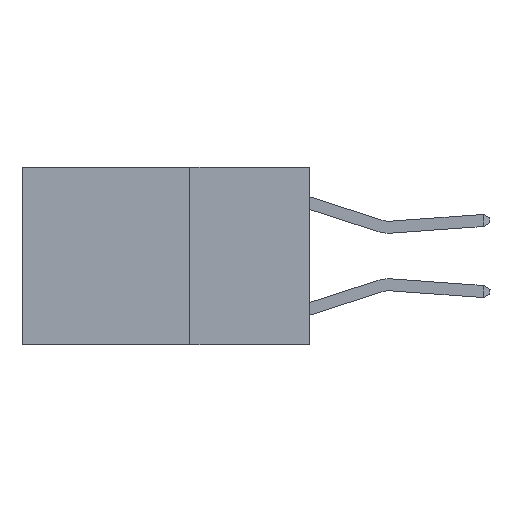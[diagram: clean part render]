
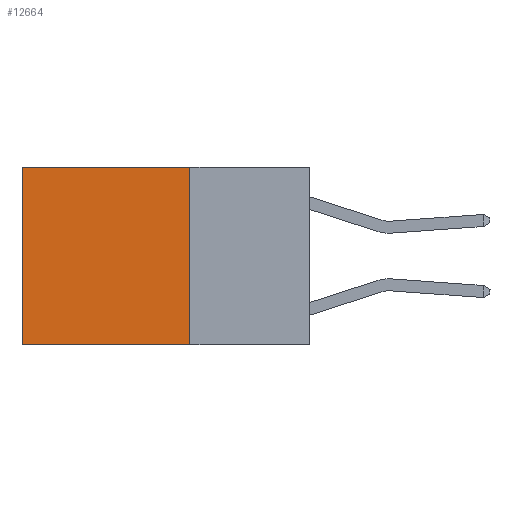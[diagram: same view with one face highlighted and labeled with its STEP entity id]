
A CAD part, left-side view. The second image highlights one B-rep face of the part: STEP entity #12664.
In plain terms, the highlighted planar face has unit normal (-1, 0, 0).
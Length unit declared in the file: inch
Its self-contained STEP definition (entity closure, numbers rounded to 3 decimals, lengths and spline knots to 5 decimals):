
#81 = CARTESIAN_POINT ( 'NONE',  ( 0.2625, 0.6, 0. ) ) ;
#1059 = DIRECTION ( 'NONE',  ( 0., 1., 0. ) ) ;
#1086 = VECTOR ( 'NONE', #16187, 39.37008 ) ;
#1292 = EDGE_CURVE ( 'NONE', #19387, #13312, #16625, .T. ) ;
#1291 = LINE ( 'NONE', #9915, #22840 ) ;
#1475 = DIRECTION ( 'NONE',  ( 1., 0., 0. ) ) ;
#2736 = CARTESIAN_POINT ( 'NONE',  ( 0.2625, 0.25, 0. ) ) ;
#3690 = LINE ( 'NONE', #7798, #1086 ) ;
#7323 = CARTESIAN_POINT ( 'NONE',  ( 0.2625, 0.6, -0.37 ) ) ;
#7798 = CARTESIAN_POINT ( 'NONE',  ( 0.2625, 0.25, 0. ) ) ;
#8352 = CARTESIAN_POINT ( 'NONE',  ( 0.2625, 0.6, 0. ) ) ;
#9445 = ORIENTED_EDGE ( 'NONE', *, *, #26035, .T. ) ;
#9915 = CARTESIAN_POINT ( 'NONE',  ( 0.2625, 0.25, -0.37 ) ) ;
#10244 = PLANE ( 'NONE',  #25109 ) ;
#12664 = ADVANCED_FACE ( 'NONE', ( #25343 ), #10244, .F. ) ;
#12784 = VECTOR ( 'NONE', #1059, 39.37008 ) ;
#12831 = EDGE_CURVE ( 'NONE', #15627, #22639, #3690, .T. ) ;
#12849 = EDGE_CURVE ( 'NONE', #22639, #13312, #1291, .T. ) ;
#13312 = VERTEX_POINT ( 'NONE', #7323 ) ;
#15627 = VERTEX_POINT ( 'NONE', #19905 ) ;
#16187 = DIRECTION ( 'NONE',  ( 0., 0., -1. ) ) ;
#16625 = LINE ( 'NONE', #8352, #18835 ) ;
#17638 = ORIENTED_EDGE ( 'NONE', *, *, #12831, .F. ) ;
#18082 = LINE ( 'NONE', #2736, #12784 ) ;
#18835 = VECTOR ( 'NONE', #21437, 39.37008 ) ;
#19387 = VERTEX_POINT ( 'NONE', #81 ) ;
#19655 = EDGE_LOOP ( 'NONE', ( #23037, #26320, #17638, #9445 ) ) ;
#19905 = CARTESIAN_POINT ( 'NONE',  ( 0.2625, 0.25, 0. ) ) ;
#21437 = DIRECTION ( 'NONE',  ( 0., 0., -1. ) ) ;
#22639 = VERTEX_POINT ( 'NONE', #24286 ) ;
#22840 = VECTOR ( 'NONE', #27279, 39.37008 ) ;
#23037 = ORIENTED_EDGE ( 'NONE', *, *, #1292, .T. ) ;
#23206 = CARTESIAN_POINT ( 'NONE',  ( 0.2625, 0.25, 0. ) ) ;
#23494 = DIRECTION ( 'NONE',  ( 0., 0., -1. ) ) ;
#24286 = CARTESIAN_POINT ( 'NONE',  ( 0.2625, 0.25, -0.37 ) ) ;
#25109 = AXIS2_PLACEMENT_3D ( 'NONE', #23206, #1475, #23494 ) ;
#25343 = FACE_OUTER_BOUND ( 'NONE', #19655, .T. ) ;
#26035 = EDGE_CURVE ( 'NONE', #15627, #19387, #18082, .T. ) ;
#26320 = ORIENTED_EDGE ( 'NONE', *, *, #12849, .F. ) ;
#27279 = DIRECTION ( 'NONE',  ( 0., 1., 0. ) ) ;
